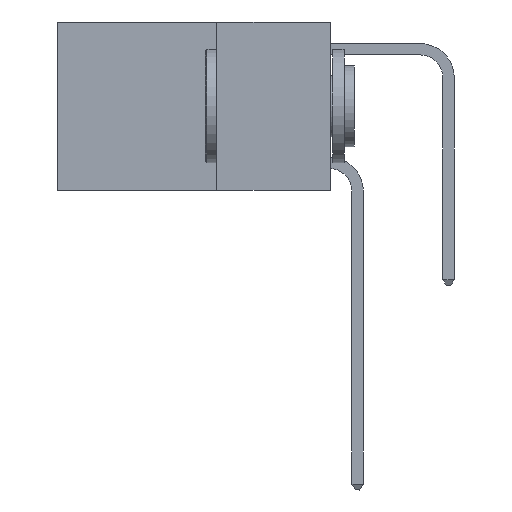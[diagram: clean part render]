
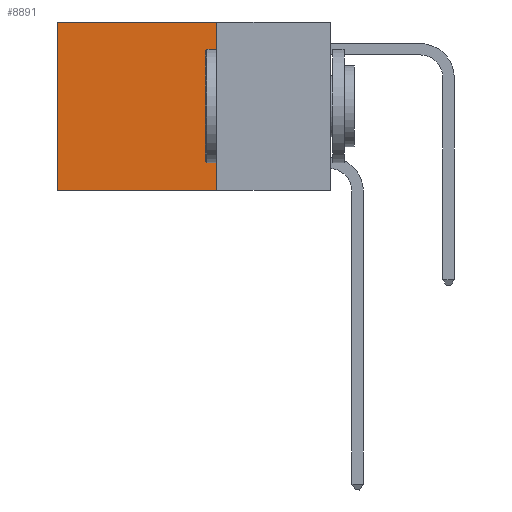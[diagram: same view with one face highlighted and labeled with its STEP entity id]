
A CAD part, left-side view. The second image highlights one B-rep face of the part: STEP entity #8891.
In plain terms, the highlighted planar face has unit normal (-1, 0, 0).
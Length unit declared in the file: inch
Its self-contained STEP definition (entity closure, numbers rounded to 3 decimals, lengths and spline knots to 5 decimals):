
#316 = LINE ( 'NONE', #6571, #8301 ) ;
#1164 = CARTESIAN_POINT ( 'NONE',  ( 0.2625, 0.6, 0. ) ) ;
#1407 = VERTEX_POINT ( 'NONE', #6097 ) ;
#1497 = VECTOR ( 'NONE', #2204, 39.37008 ) ;
#1791 = CARTESIAN_POINT ( 'NONE',  ( 0.2625, 0.6, 0. ) ) ;
#2182 = FACE_OUTER_BOUND ( 'NONE', #4232, .T. ) ;
#2204 = DIRECTION ( 'NONE',  ( 0., 0., -1. ) ) ;
#2317 = PLANE ( 'NONE',  #7155 ) ;
#2464 = CARTESIAN_POINT ( 'NONE',  ( 0.2625, 0.25, -0.37 ) ) ;
#2561 = VERTEX_POINT ( 'NONE', #1791 ) ;
#3017 = DIRECTION ( 'NONE',  ( 0., 1., 0. ) ) ;
#3449 = ORIENTED_EDGE ( 'NONE', *, *, #4968, .T. ) ;
#4104 = VECTOR ( 'NONE', #3017, 39.37008 ) ;
#4232 = EDGE_LOOP ( 'NONE', ( #3449, #7343, #12558, #9267 ) ) ;
#4345 = CARTESIAN_POINT ( 'NONE',  ( 0.2625, 0.25, 0. ) ) ;
#4968 = EDGE_CURVE ( 'NONE', #2561, #9338, #12289, .T. ) ;
#5195 = CARTESIAN_POINT ( 'NONE',  ( 0.2625, 0.25, -0.37 ) ) ;
#5379 = DIRECTION ( 'NONE',  ( 0., 0., -1. ) ) ;
#6042 = CARTESIAN_POINT ( 'NONE',  ( 0.2625, 0.25, 0. ) ) ;
#6044 = CARTESIAN_POINT ( 'NONE',  ( 0.2625, 0.6, -0.37 ) ) ;
#6097 = CARTESIAN_POINT ( 'NONE',  ( 0.2625, 0.25, 0. ) ) ;
#6571 = CARTESIAN_POINT ( 'NONE',  ( 0.2625, 0.25, 0. ) ) ;
#6575 = LINE ( 'NONE', #2464, #9111 ) ;
#6862 = LINE ( 'NONE', #6042, #4104 ) ;
#7155 = AXIS2_PLACEMENT_3D ( 'NONE', #4345, #11737, #5379 ) ;
#7343 = ORIENTED_EDGE ( 'NONE', *, *, #13225, .F. ) ;
#7487 = EDGE_CURVE ( 'NONE', #1407, #2561, #6862, .T. ) ;
#8301 = VECTOR ( 'NONE', #12971, 39.37008 ) ;
#8891 = ADVANCED_FACE ( 'NONE', ( #2182 ), #2317, .F. ) ;
#9111 = VECTOR ( 'NONE', #12988, 39.37008 ) ;
#9267 = ORIENTED_EDGE ( 'NONE', *, *, #7487, .T. ) ;
#9338 = VERTEX_POINT ( 'NONE', #6044 ) ;
#11737 = DIRECTION ( 'NONE',  ( 1., 0., 0. ) ) ;
#12046 = EDGE_CURVE ( 'NONE', #1407, #12444, #316, .T. ) ;
#12289 = LINE ( 'NONE', #1164, #1497 ) ;
#12444 = VERTEX_POINT ( 'NONE', #5195 ) ;
#12558 = ORIENTED_EDGE ( 'NONE', *, *, #12046, .F. ) ;
#12971 = DIRECTION ( 'NONE',  ( 0., 0., -1. ) ) ;
#12988 = DIRECTION ( 'NONE',  ( 0., 1., 0. ) ) ;
#13225 = EDGE_CURVE ( 'NONE', #12444, #9338, #6575, .T. ) ;
